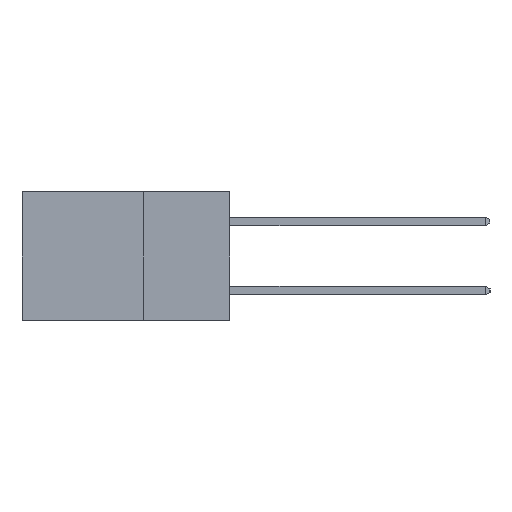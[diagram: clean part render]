
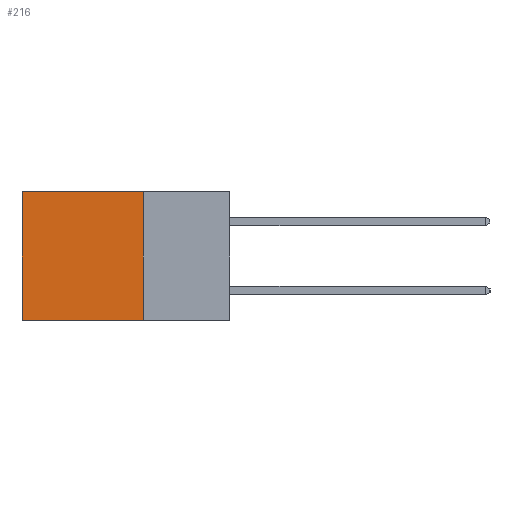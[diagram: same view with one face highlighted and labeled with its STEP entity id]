
A CAD part, left-side view. The second image highlights one B-rep face of the part: STEP entity #216.
In plain terms, the highlighted planar face has unit normal (-1, 0, 0).
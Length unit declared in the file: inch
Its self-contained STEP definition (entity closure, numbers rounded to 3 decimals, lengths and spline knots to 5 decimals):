
#216 = ADVANCED_FACE ( 'NONE', ( #4875 ), #3819, .F. ) ;
#272 = DIRECTION ( 'NONE',  ( 1., 0., 0. ) ) ;
#304 = CARTESIAN_POINT ( 'NONE',  ( 0.2615, 0.25, -0.37 ) ) ;
#497 = LINE ( 'NONE', #9942, #4795 ) ;
#515 = VECTOR ( 'NONE', #7759, 39.37008 ) ;
#1386 = CARTESIAN_POINT ( 'NONE',  ( 0.2615, 0.25, 0. ) ) ;
#1670 = VERTEX_POINT ( 'NONE', #2011 ) ;
#2011 = CARTESIAN_POINT ( 'NONE',  ( 0.2615, 0.25, 0. ) ) ;
#2105 = EDGE_LOOP ( 'NONE', ( #9770, #8862, #5428, #10310 ) ) ;
#2233 = VERTEX_POINT ( 'NONE', #5250 ) ;
#3343 = VECTOR ( 'NONE', #10602, 39.37008 ) ;
#3586 = VERTEX_POINT ( 'NONE', #10854 ) ;
#3659 = DIRECTION ( 'NONE',  ( 0., 0., -1. ) ) ;
#3819 = PLANE ( 'NONE',  #10957 ) ;
#4795 = VECTOR ( 'NONE', #3659, 39.37008 ) ;
#4870 = DIRECTION ( 'NONE',  ( 0., 0., -1. ) ) ;
#4875 = FACE_OUTER_BOUND ( 'NONE', #2105, .T. ) ;
#4995 = VERTEX_POINT ( 'NONE', #11043 ) ;
#5106 = LINE ( 'NONE', #1386, #515 ) ;
#5250 = CARTESIAN_POINT ( 'NONE',  ( 0.2615, 0.25, -0.37 ) ) ;
#5428 = ORIENTED_EDGE ( 'NONE', *, *, #7288, .F. ) ;
#7288 = EDGE_CURVE ( 'NONE', #1670, #2233, #9480, .T. ) ;
#7665 = CARTESIAN_POINT ( 'NONE',  ( 0.2615, 0.25, -0.37 ) ) ;
#7759 = DIRECTION ( 'NONE',  ( 0., 1., 0. ) ) ;
#8862 = ORIENTED_EDGE ( 'NONE', *, *, #11229, .F. ) ;
#9449 = DIRECTION ( 'NONE',  ( 0., 0., -1. ) ) ;
#9480 = LINE ( 'NONE', #7665, #11218 ) ;
#9742 = CARTESIAN_POINT ( 'NONE',  ( 0.2615, 0.25, -0.37 ) ) ;
#9770 = ORIENTED_EDGE ( 'NONE', *, *, #10738, .T. ) ;
#9878 = EDGE_CURVE ( 'NONE', #1670, #3586, #5106, .T. ) ;
#9942 = CARTESIAN_POINT ( 'NONE',  ( 0.2615, 0.6, -0.37 ) ) ;
#10310 = ORIENTED_EDGE ( 'NONE', *, *, #9878, .T. ) ;
#10465 = LINE ( 'NONE', #9742, #3343 ) ;
#10602 = DIRECTION ( 'NONE',  ( 0., 1., 0. ) ) ;
#10738 = EDGE_CURVE ( 'NONE', #3586, #4995, #497, .T. ) ;
#10854 = CARTESIAN_POINT ( 'NONE',  ( 0.2615, 0.6, 0. ) ) ;
#10957 = AXIS2_PLACEMENT_3D ( 'NONE', #304, #272, #4870 ) ;
#11043 = CARTESIAN_POINT ( 'NONE',  ( 0.2615, 0.6, -0.37 ) ) ;
#11218 = VECTOR ( 'NONE', #9449, 39.37008 ) ;
#11229 = EDGE_CURVE ( 'NONE', #2233, #4995, #10465, .T. ) ;
